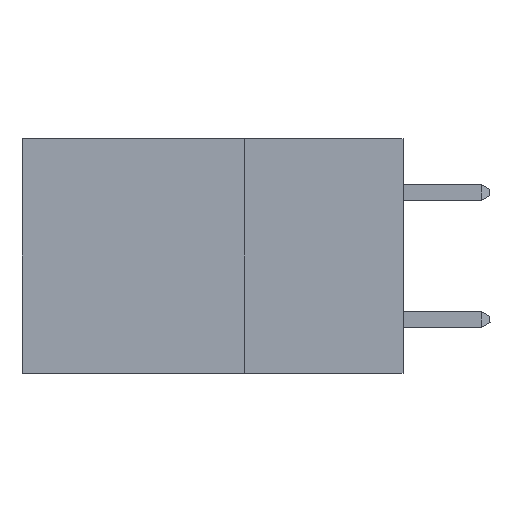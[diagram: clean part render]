
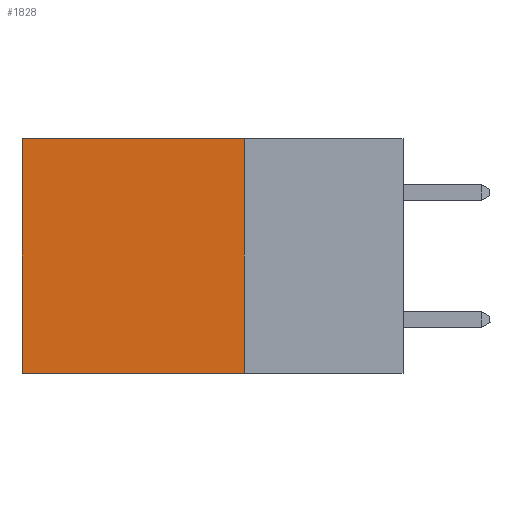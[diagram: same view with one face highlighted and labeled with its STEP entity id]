
A CAD part, left-side view. The second image highlights one B-rep face of the part: STEP entity #1828.
In plain terms, the highlighted planar face has unit normal (-1, 0, 0).
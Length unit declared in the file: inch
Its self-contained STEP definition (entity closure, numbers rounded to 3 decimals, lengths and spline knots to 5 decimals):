
#1046 = DIRECTION ( 'NONE',  ( 0., 0., -1. ) ) ;
#1223 = LINE ( 'NONE', #7547, #5369 ) ;
#1340 = VERTEX_POINT ( 'NONE', #5767 ) ;
#1828 = ADVANCED_FACE ( 'NONE', ( #9955 ), #4029, .F. ) ;
#2198 = VERTEX_POINT ( 'NONE', #9617 ) ;
#2678 = EDGE_CURVE ( 'NONE', #5396, #2198, #8696, .T. ) ;
#3038 = VERTEX_POINT ( 'NONE', #3941 ) ;
#3043 = DIRECTION ( 'NONE',  ( 1., 0., 0. ) ) ;
#3472 = CARTESIAN_POINT ( 'NONE',  ( 0.2875, 0.25, 0. ) ) ;
#3684 = ORIENTED_EDGE ( 'NONE', *, *, #6611, .F. ) ;
#3941 = CARTESIAN_POINT ( 'NONE',  ( 0.2875, 0.6, 0. ) ) ;
#4029 = PLANE ( 'NONE',  #5701 ) ;
#4611 = ORIENTED_EDGE ( 'NONE', *, *, #8823, .T. ) ;
#4614 = VECTOR ( 'NONE', #5477, 39.37008 ) ;
#5075 = ORIENTED_EDGE ( 'NONE', *, *, #5819, .T. ) ;
#5369 = VECTOR ( 'NONE', #9228, 39.37008 ) ;
#5396 = VERTEX_POINT ( 'NONE', #8243 ) ;
#5471 = CARTESIAN_POINT ( 'NONE',  ( 0.2875, 0.6, 0. ) ) ;
#5477 = DIRECTION ( 'NONE',  ( 0., 1., 0. ) ) ;
#5701 = AXIS2_PLACEMENT_3D ( 'NONE', #7463, #3043, #6709 ) ;
#5767 = CARTESIAN_POINT ( 'NONE',  ( 0.2875, 0.25, 0. ) ) ;
#5819 = EDGE_CURVE ( 'NONE', #1340, #3038, #9846, .T. ) ;
#6611 = EDGE_CURVE ( 'NONE', #1340, #5396, #1223, .T. ) ;
#6659 = CARTESIAN_POINT ( 'NONE',  ( 0.2875, 0.25, -0.37 ) ) ;
#6709 = DIRECTION ( 'NONE',  ( 0., 0., -1. ) ) ;
#7463 = CARTESIAN_POINT ( 'NONE',  ( 0.2875, 0.25, 0. ) ) ;
#7547 = CARTESIAN_POINT ( 'NONE',  ( 0.2875, 0.25, 0. ) ) ;
#7860 = ORIENTED_EDGE ( 'NONE', *, *, #2678, .F. ) ;
#8243 = CARTESIAN_POINT ( 'NONE',  ( 0.2875, 0.25, -0.37 ) ) ;
#8696 = LINE ( 'NONE', #6659, #10374 ) ;
#8823 = EDGE_CURVE ( 'NONE', #3038, #2198, #10240, .T. ) ;
#9093 = DIRECTION ( 'NONE',  ( 0., 1., 0. ) ) ;
#9187 = EDGE_LOOP ( 'NONE', ( #4611, #7860, #3684, #5075 ) ) ;
#9228 = DIRECTION ( 'NONE',  ( 0., 0., -1. ) ) ;
#9617 = CARTESIAN_POINT ( 'NONE',  ( 0.2875, 0.6, -0.37 ) ) ;
#9670 = VECTOR ( 'NONE', #1046, 39.37008 ) ;
#9846 = LINE ( 'NONE', #3472, #4614 ) ;
#9955 = FACE_OUTER_BOUND ( 'NONE', #9187, .T. ) ;
#10240 = LINE ( 'NONE', #5471, #9670 ) ;
#10374 = VECTOR ( 'NONE', #9093, 39.37008 ) ;
